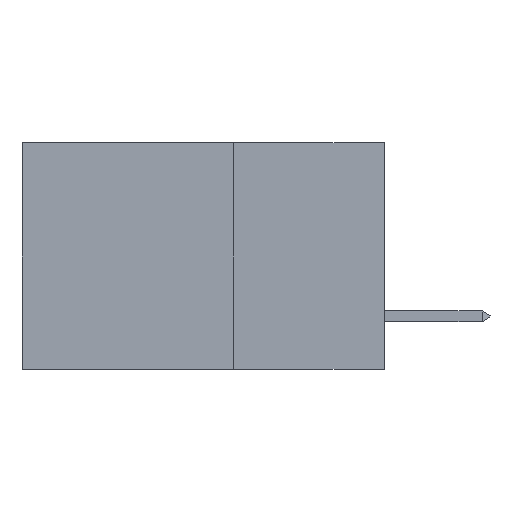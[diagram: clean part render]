
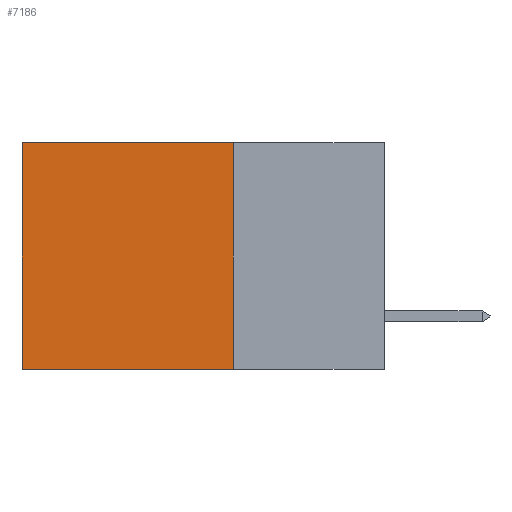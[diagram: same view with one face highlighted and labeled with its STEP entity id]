
A CAD part, left-side view. The second image highlights one B-rep face of the part: STEP entity #7186.
In plain terms, the highlighted planar face has unit normal (-1, 0, 0).
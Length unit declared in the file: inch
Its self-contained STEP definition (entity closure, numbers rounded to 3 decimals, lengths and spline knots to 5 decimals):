
#271 = EDGE_CURVE ( 'NONE', #5604, #5614, #9020, .T. ) ;
#864 = EDGE_LOOP ( 'NONE', ( #9732, #3841, #4668, #7266 ) ) ;
#2531 = CARTESIAN_POINT ( 'NONE',  ( 0.2875, 0.25, -0.375 ) ) ;
#2681 = DIRECTION ( 'NONE',  ( 1., 0., 0. ) ) ;
#2732 = CARTESIAN_POINT ( 'NONE',  ( 0.2875, 0.25, -0.375 ) ) ;
#3205 = CARTESIAN_POINT ( 'NONE',  ( 0.2875, 0.6, -0.375 ) ) ;
#3409 = VECTOR ( 'NONE', #4491, 39.37008 ) ;
#3841 = ORIENTED_EDGE ( 'NONE', *, *, #6215, .F. ) ;
#4491 = DIRECTION ( 'NONE',  ( 0., 0., -1. ) ) ;
#4668 = ORIENTED_EDGE ( 'NONE', *, *, #15642, .F. ) ;
#4840 = CARTESIAN_POINT ( 'NONE',  ( 0.2875, 0.25, -0.375 ) ) ;
#5604 = VERTEX_POINT ( 'NONE', #12410 ) ;
#5614 = VERTEX_POINT ( 'NONE', #10767 ) ;
#5851 = FACE_OUTER_BOUND ( 'NONE', #864, .T. ) ;
#5899 = LINE ( 'NONE', #4840, #8290 ) ;
#6040 = LINE ( 'NONE', #7678, #15743 ) ;
#6215 = EDGE_CURVE ( 'NONE', #11087, #5614, #5899, .T. ) ;
#6583 = DIRECTION ( 'NONE',  ( 0., 0., -1. ) ) ;
#7186 = ADVANCED_FACE ( 'NONE', ( #5851 ), #9045, .F. ) ;
#7266 = ORIENTED_EDGE ( 'NONE', *, *, #9395, .T. ) ;
#7678 = CARTESIAN_POINT ( 'NONE',  ( 0.2875, 0.25, -0.375 ) ) ;
#7841 = DIRECTION ( 'NONE',  ( 0., 1., 0. ) ) ;
#8290 = VECTOR ( 'NONE', #12390, 39.37008 ) ;
#9020 = LINE ( 'NONE', #3205, #3409 ) ;
#9045 = PLANE ( 'NONE',  #11378 ) ;
#9395 = EDGE_CURVE ( 'NONE', #12355, #5604, #14118, .T. ) ;
#9732 = ORIENTED_EDGE ( 'NONE', *, *, #271, .T. ) ;
#10767 = CARTESIAN_POINT ( 'NONE',  ( 0.2875, 0.6, -0.375 ) ) ;
#11087 = VERTEX_POINT ( 'NONE', #2531 ) ;
#11378 = AXIS2_PLACEMENT_3D ( 'NONE', #2732, #2681, #6583 ) ;
#11674 = CARTESIAN_POINT ( 'NONE',  ( 0.2875, 0.25, 0. ) ) ;
#12355 = VERTEX_POINT ( 'NONE', #13671 ) ;
#12390 = DIRECTION ( 'NONE',  ( 0., 1., 0. ) ) ;
#12410 = CARTESIAN_POINT ( 'NONE',  ( 0.2875, 0.6, 0. ) ) ;
#12727 = DIRECTION ( 'NONE',  ( 0., 0., -1. ) ) ;
#13671 = CARTESIAN_POINT ( 'NONE',  ( 0.2875, 0.25, 0. ) ) ;
#13910 = VECTOR ( 'NONE', #7841, 39.37008 ) ;
#14118 = LINE ( 'NONE', #11674, #13910 ) ;
#15642 = EDGE_CURVE ( 'NONE', #12355, #11087, #6040, .T. ) ;
#15743 = VECTOR ( 'NONE', #12727, 39.37008 ) ;
